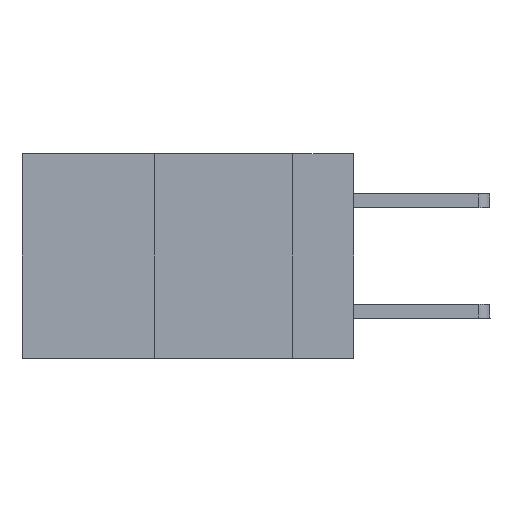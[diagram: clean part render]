
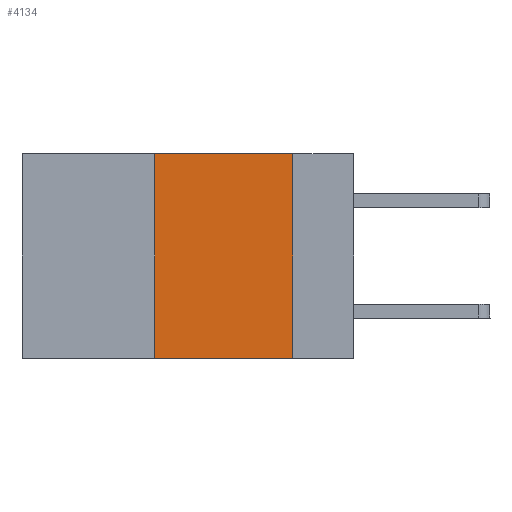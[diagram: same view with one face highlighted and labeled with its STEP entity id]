
A CAD part, left-side view. The second image highlights one B-rep face of the part: STEP entity #4134.
In plain terms, the highlighted planar face has unit normal (-1, 0, 0).
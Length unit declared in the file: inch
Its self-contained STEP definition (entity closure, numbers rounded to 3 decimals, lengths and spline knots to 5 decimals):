
#171 = VECTOR ( 'NONE', #4344, 39.37008 ) ;
#213 = VERTEX_POINT ( 'NONE', #4293 ) ;
#407 = VERTEX_POINT ( 'NONE', #3635 ) ;
#1349 = LINE ( 'NONE', #4448, #10137 ) ;
#1735 = CARTESIAN_POINT ( 'NONE',  ( 0., 0.11, 0. ) ) ;
#1753 = EDGE_CURVE ( 'NONE', #407, #10592, #9907, .T. ) ;
#2140 = DIRECTION ( 'NONE',  ( 0., 0., -1. ) ) ;
#2237 = CARTESIAN_POINT ( 'NONE',  ( 0., 0.11, 0. ) ) ;
#3084 = CARTESIAN_POINT ( 'NONE',  ( 0., 0.6, 0. ) ) ;
#3124 = DIRECTION ( 'NONE',  ( 0., -1., 0. ) ) ;
#3296 = CARTESIAN_POINT ( 'NONE',  ( 0., 0.6, -0.37 ) ) ;
#3635 = CARTESIAN_POINT ( 'NONE',  ( 0., 0.36, 0. ) ) ;
#4134 = ADVANCED_FACE ( 'NONE', ( #9461 ), #9871, .F. ) ;
#4293 = CARTESIAN_POINT ( 'NONE',  ( 0., 0.36, -0.37 ) ) ;
#4344 = DIRECTION ( 'NONE',  ( 0., -1., 0. ) ) ;
#4376 = VECTOR ( 'NONE', #2140, 39.37008 ) ;
#4448 = CARTESIAN_POINT ( 'NONE',  ( 0., 0.36, 0. ) ) ;
#5206 = EDGE_CURVE ( 'NONE', #10592, #6072, #11524, .T. ) ;
#5563 = VECTOR ( 'NONE', #3124, 39.37008 ) ;
#5969 = AXIS2_PLACEMENT_3D ( 'NONE', #10106, #9849, #9847 ) ;
#6072 = VERTEX_POINT ( 'NONE', #7515 ) ;
#6805 = EDGE_LOOP ( 'NONE', ( #10147, #10118, #10195, #10167 ) ) ;
#7515 = CARTESIAN_POINT ( 'NONE',  ( 0., 0.11, -0.37 ) ) ;
#7687 = EDGE_CURVE ( 'NONE', #213, #407, #1349, .T. ) ;
#9461 = FACE_OUTER_BOUND ( 'NONE', #6805, .T. ) ;
#9789 = DIRECTION ( 'NONE',  ( 0., 0., 1. ) ) ;
#9847 = DIRECTION ( 'NONE',  ( 0., 0., -1. ) ) ;
#9849 = DIRECTION ( 'NONE',  ( 1., 0., 0. ) ) ;
#9871 = PLANE ( 'NONE',  #5969 ) ;
#9907 = LINE ( 'NONE', #3084, #5563 ) ;
#10106 = CARTESIAN_POINT ( 'NONE',  ( 0., 0.6, 0. ) ) ;
#10118 = ORIENTED_EDGE ( 'NONE', *, *, #1753, .F. ) ;
#10137 = VECTOR ( 'NONE', #9789, 39.37008 ) ;
#10147 = ORIENTED_EDGE ( 'NONE', *, *, #5206, .F. ) ;
#10164 = LINE ( 'NONE', #3296, #171 ) ;
#10167 = ORIENTED_EDGE ( 'NONE', *, *, #10362, .T. ) ;
#10195 = ORIENTED_EDGE ( 'NONE', *, *, #7687, .F. ) ;
#10362 = EDGE_CURVE ( 'NONE', #213, #6072, #10164, .T. ) ;
#10592 = VERTEX_POINT ( 'NONE', #1735 ) ;
#11524 = LINE ( 'NONE', #2237, #4376 ) ;
